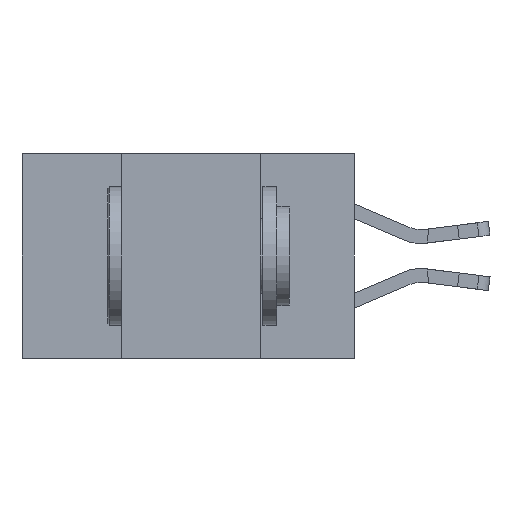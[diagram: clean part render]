
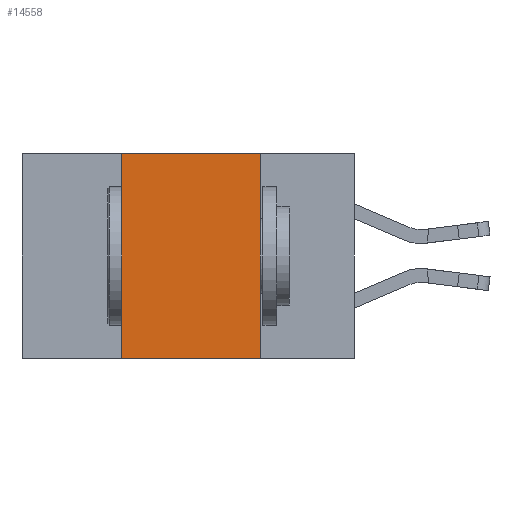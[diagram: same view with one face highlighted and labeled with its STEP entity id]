
A CAD part, left-side view. The second image highlights one B-rep face of the part: STEP entity #14558.
In plain terms, the highlighted planar face has unit normal (-1, 0, 0).
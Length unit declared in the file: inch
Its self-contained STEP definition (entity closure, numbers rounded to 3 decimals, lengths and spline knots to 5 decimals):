
#9 = DIRECTION ( 'NONE',  ( 0., -1., 0. ) ) ;
#153 = ORIENTED_EDGE ( 'NONE', *, *, #15269, .F. ) ;
#413 = DIRECTION ( 'NONE',  ( 0., 0., 1. ) ) ;
#497 = CARTESIAN_POINT ( 'NONE',  ( 0., 0.17, 0. ) ) ;
#2929 = EDGE_LOOP ( 'NONE', ( #6846, #153, #10988, #12933 ) ) ;
#3420 = VECTOR ( 'NONE', #6317, 39.37008 ) ;
#4705 = DIRECTION ( 'NONE',  ( 1., 0., 0. ) ) ;
#4935 = VERTEX_POINT ( 'NONE', #15342 ) ;
#5487 = CARTESIAN_POINT ( 'NONE',  ( 0., 0.17, 0. ) ) ;
#5488 = LINE ( 'NONE', #15445, #15502 ) ;
#5555 = EDGE_CURVE ( 'NONE', #4935, #14920, #9102, .T. ) ;
#6317 = DIRECTION ( 'NONE',  ( 0., -1., 0. ) ) ;
#6846 = ORIENTED_EDGE ( 'NONE', *, *, #7232, .F. ) ;
#6878 = PLANE ( 'NONE',  #13162 ) ;
#6907 = VECTOR ( 'NONE', #413, 39.37008 ) ;
#7232 = EDGE_CURVE ( 'NONE', #16300, #14920, #10076, .T. ) ;
#7432 = CARTESIAN_POINT ( 'NONE',  ( 0., 0.6, 0. ) ) ;
#7816 = CARTESIAN_POINT ( 'NONE',  ( 0., 0.6, -0.37 ) ) ;
#8247 = CARTESIAN_POINT ( 'NONE',  ( 0., 0.42, 0. ) ) ;
#8660 = CARTESIAN_POINT ( 'NONE',  ( 0., 0.17, -0.37 ) ) ;
#9102 = LINE ( 'NONE', #7816, #3420 ) ;
#9301 = VERTEX_POINT ( 'NONE', #12137 ) ;
#10076 = LINE ( 'NONE', #5487, #15821 ) ;
#10141 = FACE_OUTER_BOUND ( 'NONE', #2929, .T. ) ;
#10988 = ORIENTED_EDGE ( 'NONE', *, *, #15079, .F. ) ;
#12137 = CARTESIAN_POINT ( 'NONE',  ( 0., 0.42, 0. ) ) ;
#12933 = ORIENTED_EDGE ( 'NONE', *, *, #5555, .T. ) ;
#13162 = AXIS2_PLACEMENT_3D ( 'NONE', #7432, #4705, #16571 ) ;
#13457 = DIRECTION ( 'NONE',  ( 0., 0., -1. ) ) ;
#14558 = ADVANCED_FACE ( 'NONE', ( #10141 ), #6878, .F. ) ;
#14920 = VERTEX_POINT ( 'NONE', #8660 ) ;
#15079 = EDGE_CURVE ( 'NONE', #4935, #9301, #16141, .T. ) ;
#15269 = EDGE_CURVE ( 'NONE', #9301, #16300, #5488, .T. ) ;
#15342 = CARTESIAN_POINT ( 'NONE',  ( 0., 0.42, -0.37 ) ) ;
#15445 = CARTESIAN_POINT ( 'NONE',  ( 0., 0.6, 0. ) ) ;
#15502 = VECTOR ( 'NONE', #9, 39.37008 ) ;
#15821 = VECTOR ( 'NONE', #13457, 39.37008 ) ;
#16141 = LINE ( 'NONE', #8247, #6907 ) ;
#16300 = VERTEX_POINT ( 'NONE', #497 ) ;
#16571 = DIRECTION ( 'NONE',  ( 0., 0., -1. ) ) ;
